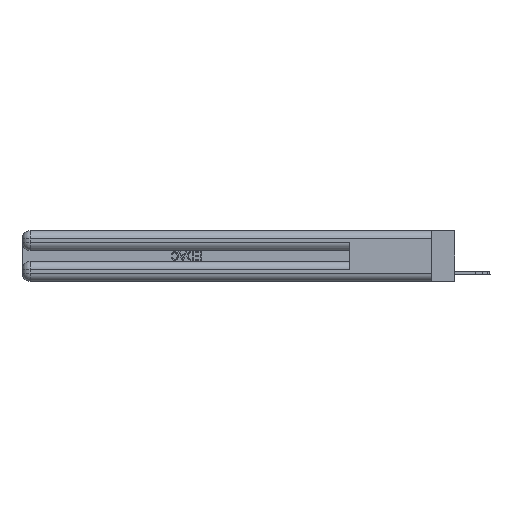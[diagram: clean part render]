
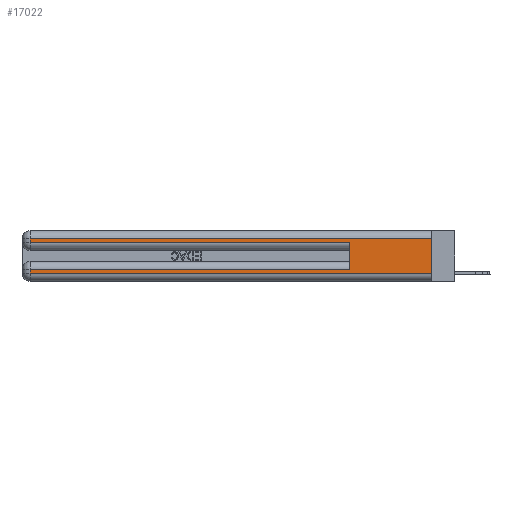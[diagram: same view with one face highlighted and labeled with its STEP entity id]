
A CAD part, left-side view. The second image highlights one B-rep face of the part: STEP entity #17022.
In plain terms, the highlighted planar face has unit normal (-1, 0, 0).
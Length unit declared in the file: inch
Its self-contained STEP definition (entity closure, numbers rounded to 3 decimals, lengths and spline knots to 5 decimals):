
#221 = ORIENTED_EDGE ( 'NONE', *, *, #19243, .F. ) ;
#529 = DIRECTION ( 'NONE',  ( 0., 0., -1. ) ) ;
#1838 = ORIENTED_EDGE ( 'NONE', *, *, #14964, .F. ) ;
#1847 = AXIS2_PLACEMENT_3D ( 'NONE', #18438, #21267, #529 ) ;
#2597 = CARTESIAN_POINT ( 'NONE',  ( 0., 0., 0.37 ) ) ;
#2598 = EDGE_CURVE ( 'NONE', #14537, #11547, #13773, .T. ) ;
#2751 = DIRECTION ( 'NONE',  ( 0., 0., -1. ) ) ;
#2781 = FACE_OUTER_BOUND ( 'NONE', #29726, .T. ) ;
#3314 = CARTESIAN_POINT ( 'NONE',  ( 0., 2.94, 0.31 ) ) ;
#3747 = VECTOR ( 'NONE', #16200, 39.37008 ) ;
#4771 = VECTOR ( 'NONE', #23646, 39.37008 ) ;
#5107 = VERTEX_POINT ( 'NONE', #3314 ) ;
#6350 = CARTESIAN_POINT ( 'NONE',  ( 0., 0.6, 0.085 ) ) ;
#7184 = VECTOR ( 'NONE', #11956, 39.37008 ) ;
#7307 = CARTESIAN_POINT ( 'NONE',  ( 0., 2.94, 0.37 ) ) ;
#7481 = EDGE_CURVE ( 'NONE', #12709, #20768, #14267, .T. ) ;
#8211 = CARTESIAN_POINT ( 'NONE',  ( 0., 0.6, 0.285 ) ) ;
#8524 = VECTOR ( 'NONE', #29072, 39.37008 ) ;
#9040 = VECTOR ( 'NONE', #20940, 39.37008 ) ;
#10207 = VECTOR ( 'NONE', #25684, 39.37008 ) ;
#10297 = ORIENTED_EDGE ( 'NONE', *, *, #19972, .T. ) ;
#11547 = VERTEX_POINT ( 'NONE', #8211 ) ;
#11800 = CARTESIAN_POINT ( 'NONE',  ( 0., 0., 0.06 ) ) ;
#11956 = DIRECTION ( 'NONE',  ( 0., -1., 0. ) ) ;
#12051 = CARTESIAN_POINT ( 'NONE',  ( 0., 2.94, 0.37 ) ) ;
#12066 = PLANE ( 'NONE',  #1847 ) ;
#12709 = VERTEX_POINT ( 'NONE', #24638 ) ;
#13773 = LINE ( 'NONE', #13930, #3747 ) ;
#13930 = CARTESIAN_POINT ( 'NONE',  ( 0., 0., 0.285 ) ) ;
#14267 = LINE ( 'NONE', #7307, #10207 ) ;
#14474 = CARTESIAN_POINT ( 'NONE',  ( 0., 0., 0.085 ) ) ;
#14537 = VERTEX_POINT ( 'NONE', #15931 ) ;
#14964 = EDGE_CURVE ( 'NONE', #23005, #20617, #18988, .T. ) ;
#15931 = CARTESIAN_POINT ( 'NONE',  ( 0., 2.94, 0.285 ) ) ;
#15974 = ORIENTED_EDGE ( 'NONE', *, *, #21410, .T. ) ;
#16042 = ORIENTED_EDGE ( 'NONE', *, *, #26460, .T. ) ;
#16200 = DIRECTION ( 'NONE',  ( 0., -1., 0. ) ) ;
#17022 = ADVANCED_FACE ( 'NONE', ( #2781 ), #12066, .F. ) ;
#17472 = LINE ( 'NONE', #28989, #26662 ) ;
#17611 = DIRECTION ( 'NONE',  ( 0., 1., 0. ) ) ;
#17862 = EDGE_CURVE ( 'NONE', #20768, #20617, #20999, .T. ) ;
#18001 = CARTESIAN_POINT ( 'NONE',  ( 0., 0., 0.06 ) ) ;
#18438 = CARTESIAN_POINT ( 'NONE',  ( 0., 0., 0.37 ) ) ;
#18988 = LINE ( 'NONE', #2597, #21108 ) ;
#19243 = EDGE_CURVE ( 'NONE', #29279, #11547, #19970, .T. ) ;
#19877 = ORIENTED_EDGE ( 'NONE', *, *, #7481, .T. ) ;
#19946 = ORIENTED_EDGE ( 'NONE', *, *, #2598, .T. ) ;
#19970 = LINE ( 'NONE', #22660, #8524 ) ;
#19972 = EDGE_CURVE ( 'NONE', #5107, #14537, #25882, .T. ) ;
#20617 = VERTEX_POINT ( 'NONE', #18001 ) ;
#20768 = VERTEX_POINT ( 'NONE', #25334 ) ;
#20940 = DIRECTION ( 'NONE',  ( 0., 0., -1. ) ) ;
#20999 = LINE ( 'NONE', #11800, #7184 ) ;
#21108 = VECTOR ( 'NONE', #2751, 39.37008 ) ;
#21267 = DIRECTION ( 'NONE',  ( 1., 0., 0. ) ) ;
#21410 = EDGE_CURVE ( 'NONE', #29279, #12709, #25887, .T. ) ;
#21509 = CARTESIAN_POINT ( 'NONE',  ( 0., 0., 0.31 ) ) ;
#22660 = CARTESIAN_POINT ( 'NONE',  ( 0., 0.6, 0.145 ) ) ;
#23005 = VERTEX_POINT ( 'NONE', #21509 ) ;
#23646 = DIRECTION ( 'NONE',  ( 0., 1., 0. ) ) ;
#24638 = CARTESIAN_POINT ( 'NONE',  ( 0., 2.94, 0.085 ) ) ;
#25334 = CARTESIAN_POINT ( 'NONE',  ( 0., 2.94, 0.06 ) ) ;
#25684 = DIRECTION ( 'NONE',  ( 0., 0., -1. ) ) ;
#25882 = LINE ( 'NONE', #12051, #9040 ) ;
#25887 = LINE ( 'NONE', #14474, #4771 ) ;
#26460 = EDGE_CURVE ( 'NONE', #23005, #5107, #17472, .T. ) ;
#26662 = VECTOR ( 'NONE', #17611, 39.37008 ) ;
#28949 = ORIENTED_EDGE ( 'NONE', *, *, #17862, .T. ) ;
#28989 = CARTESIAN_POINT ( 'NONE',  ( 0., 0., 0.31 ) ) ;
#29072 = DIRECTION ( 'NONE',  ( 0., 0., 1. ) ) ;
#29279 = VERTEX_POINT ( 'NONE', #6350 ) ;
#29726 = EDGE_LOOP ( 'NONE', ( #1838, #16042, #10297, #19946, #221, #15974, #19877, #28949 ) ) ;
